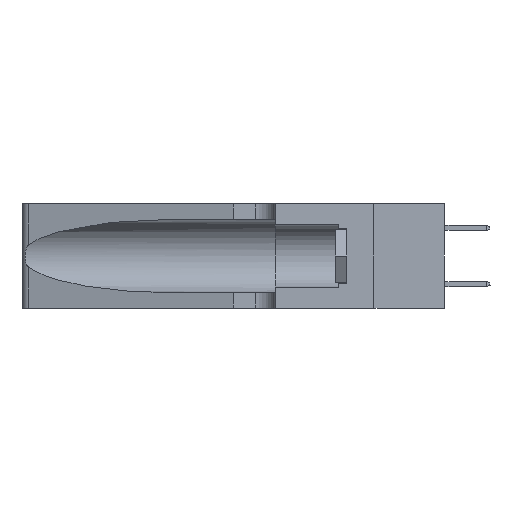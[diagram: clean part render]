
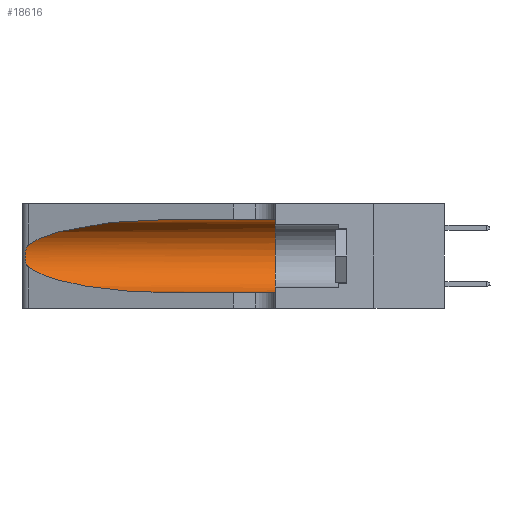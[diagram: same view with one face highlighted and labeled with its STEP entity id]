
A CAD part, left-side view. The second image highlights one B-rep face of the part: STEP entity #18616.
In plain terms, the highlighted cylindrical face has radius 3.308 mm (diameter 6.617 mm), a partial arc.
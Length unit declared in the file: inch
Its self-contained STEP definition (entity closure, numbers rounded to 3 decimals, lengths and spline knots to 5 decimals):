
#225 = CARTESIAN_POINT ( 'NONE',  ( 0.26017, 1.23833, 0.17102 ) ) ;
#260 = CARTESIAN_POINT ( 'NONE',  ( 0.25487, 1.22718, 0.14631 ) ) ;
#2554 = CARTESIAN_POINT ( 'NONE',  ( 0.1305, 0.35, 0.31525 ) ) ;
#2792 = CARTESIAN_POINT ( 'NONE',  ( 0.25639, 1.23186, 0.15144 ) ) ;
#3074 = CARTESIAN_POINT ( 'NONE',  ( 0.1305, 0.72297, 0.05475 ) ) ;
#3121 = CARTESIAN_POINT ( 'NONE',  ( 0.25487, 1.22718, 0.22369 ) ) ;
#4202 = CYLINDRICAL_SURFACE ( 'NONE', #16849, 0.13025 ) ;
#4427 = ORIENTED_EDGE ( 'NONE', *, *, #19745, .T. ) ;
#5172 = CARTESIAN_POINT ( 'NONE',  ( 0.1305, 1.61858, 0.185 ) ) ;
#5225 = EDGE_CURVE ( 'NONE', #17321, #27886, #22845, .T. ) ;
#5380 = FACE_OUTER_BOUND ( 'NONE', #14193, .T. ) ;
#5615 = B_SPLINE_CURVE_WITH_KNOTS ( 'NONE', 3,
 ( #3121, #21396, #26305, #10499, #28834, #13185, #31558, #26505, #225, #21080, #31771, #2792, #16137, #23990 ),
 .UNSPECIFIED., .F., .F.,
 ( 4, 2, 2, 2, 2, 2, 4 ),
 ( 0., 0.00027, 0.00053, 0.00107, 0.0016, 0.00187, 0.00214 ),
 .UNSPECIFIED. ) ;
#6025 = ORIENTED_EDGE ( 'NONE', *, *, #33415, .T. ) ;
#6818 = DIRECTION ( 'NONE',  ( 0., 0., -1. ) ) ;
#7899 = VECTOR ( 'NONE', #11919, 39.37008 ) ;
#10499 = CARTESIAN_POINT ( 'NONE',  ( 0.25787, 1.23484, 0.2124 ) ) ;
#10959 = ORIENTED_EDGE ( 'NONE', *, *, #17367, .T. ) ;
#11108 = CARTESIAN_POINT ( 'NONE',  ( 0.1305, 0.72297, 0.31525 ) ) ;
#11328 = VERTEX_POINT ( 'NONE', #22245 ) ;
#11531 = LINE ( 'NONE', #24931, #7899 ) ;
#11566 = DIRECTION ( 'NONE',  ( 0., 0., 1. ) ) ;
#11773 = ORIENTED_EDGE ( 'NONE', *, *, #5225, .F. ) ;
#11913 = EDGE_CURVE ( 'NONE', #22708, #27886, #13933, .T. ) ;
#11919 = DIRECTION ( 'NONE',  ( 0., -1., 0. ) ) ;
#12968 = VERTEX_POINT ( 'NONE', #19951 ) ;
#13185 = CARTESIAN_POINT ( 'NONE',  ( 0.26018, 1.23835, 0.19895 ) ) ;
#13933 = LINE ( 'NONE', #32049, #31911 ) ;
#13958 = CARTESIAN_POINT ( 'NONE',  ( 0.1305, 0.72297, 0.05475 ) ) ;
#14193 = EDGE_LOOP ( 'NONE', ( #4427, #6025, #10959, #30025, #11773, #33253 ) ) ;
#16137 = CARTESIAN_POINT ( 'NONE',  ( 0.25555, 1.22993, 0.14849 ) ) ;
#16849 = AXIS2_PLACEMENT_3D ( 'NONE', #5172, #21329, #6818 ) ;
#17169 = AXIS2_PLACEMENT_3D ( 'NONE', #29604, #28185, #11566 ) ;
#17321 = VERTEX_POINT ( 'NONE', #2554 ) ;
#17367 = EDGE_CURVE ( 'NONE', #24137, #22708, #29952, .T. ) ;
#17903 =( BOUNDED_CURVE ( )  B_SPLINE_CURVE ( 3, ( #11108, #23856, #25216, #21776 ),
 .UNSPECIFIED., .F., .T. ) 
 B_SPLINE_CURVE_WITH_KNOTS ( ( 4, 4 ),
 ( 1.5708, 2.84003 ),
 .UNSPECIFIED. ) 
 CURVE ( )  GEOMETRIC_REPRESENTATION_ITEM ( )  RATIONAL_B_SPLINE_CURVE ( ( 1., 0.87, 0.87, 1. ) ) 
 REPRESENTATION_ITEM ( '' )  );
#18616 = ADVANCED_FACE ( 'NONE', ( #5380 ), #4202, .F. ) ;
#19745 = EDGE_CURVE ( 'NONE', #12968, #11328, #17903, .T. ) ;
#19951 = CARTESIAN_POINT ( 'NONE',  ( 0.1305, 0.72297, 0.31525 ) ) ;
#20920 = CARTESIAN_POINT ( 'NONE',  ( 0.2373, 1.15595, 0.08982 ) ) ;
#21080 = CARTESIAN_POINT ( 'NONE',  ( 0.25856, 1.23593, 0.16098 ) ) ;
#21329 = DIRECTION ( 'NONE',  ( 0., -1., 0. ) ) ;
#21396 = CARTESIAN_POINT ( 'NONE',  ( 0.25555, 1.22994, 0.2215 ) ) ;
#21776 = CARTESIAN_POINT ( 'NONE',  ( 0.25487, 1.22718, 0.22369 ) ) ;
#22245 = CARTESIAN_POINT ( 'NONE',  ( 0.25487, 1.22718, 0.22369 ) ) ;
#22708 = VERTEX_POINT ( 'NONE', #13958 ) ;
#22845 = CIRCLE ( 'NONE', #17169, 0.13025 ) ;
#23430 = CARTESIAN_POINT ( 'NONE',  ( 0.25487, 1.22718, 0.14631 ) ) ;
#23856 = CARTESIAN_POINT ( 'NONE',  ( 0.18966, 0.96281, 0.31525 ) ) ;
#23990 = CARTESIAN_POINT ( 'NONE',  ( 0.25487, 1.22718, 0.14631 ) ) ;
#24137 = VERTEX_POINT ( 'NONE', #260 ) ;
#24931 = CARTESIAN_POINT ( 'NONE',  ( 0.1305, 1.61858, 0.31525 ) ) ;
#25216 = CARTESIAN_POINT ( 'NONE',  ( 0.2373, 1.15595, 0.28018 ) ) ;
#26253 = CARTESIAN_POINT ( 'NONE',  ( 0.18966, 0.96281, 0.05475 ) ) ;
#26305 = CARTESIAN_POINT ( 'NONE',  ( 0.25639, 1.23184, 0.21858 ) ) ;
#26505 = CARTESIAN_POINT ( 'NONE',  ( 0.26075, 1.23896, 0.178 ) ) ;
#27013 = DIRECTION ( 'NONE',  ( 0., -1., 0. ) ) ;
#27886 = VERTEX_POINT ( 'NONE', #29408 ) ;
#28060 = EDGE_CURVE ( 'NONE', #12968, #17321, #11531, .T. ) ;
#28185 = DIRECTION ( 'NONE',  ( 0., 1., 0. ) ) ;
#28834 = CARTESIAN_POINT ( 'NONE',  ( 0.25854, 1.2359, 0.20912 ) ) ;
#29408 = CARTESIAN_POINT ( 'NONE',  ( 0.1305, 0.35, 0.05475 ) ) ;
#29604 = CARTESIAN_POINT ( 'NONE',  ( 0.1305, 0.35, 0.185 ) ) ;
#29952 =( BOUNDED_CURVE ( )  B_SPLINE_CURVE ( 3, ( #23430, #20920, #26253, #3074 ),
 .UNSPECIFIED., .F., .F. ) 
 B_SPLINE_CURVE_WITH_KNOTS ( ( 4, 4 ),
 ( 3.44316, 4.71239 ),
 .UNSPECIFIED. ) 
 CURVE ( )  GEOMETRIC_REPRESENTATION_ITEM ( )  RATIONAL_B_SPLINE_CURVE ( ( 1., 0.87, 0.87, 1. ) ) 
 REPRESENTATION_ITEM ( '' )  );
#30025 = ORIENTED_EDGE ( 'NONE', *, *, #11913, .T. ) ;
#31558 = CARTESIAN_POINT ( 'NONE',  ( 0.26075, 1.23896, 0.19203 ) ) ;
#31771 = CARTESIAN_POINT ( 'NONE',  ( 0.25789, 1.23486, 0.15765 ) ) ;
#31911 = VECTOR ( 'NONE', #27013, 39.37008 ) ;
#32049 = CARTESIAN_POINT ( 'NONE',  ( 0.1305, 1.61858, 0.05475 ) ) ;
#33253 = ORIENTED_EDGE ( 'NONE', *, *, #28060, .F. ) ;
#33415 = EDGE_CURVE ( 'NONE', #11328, #24137, #5615, .T. ) ;
